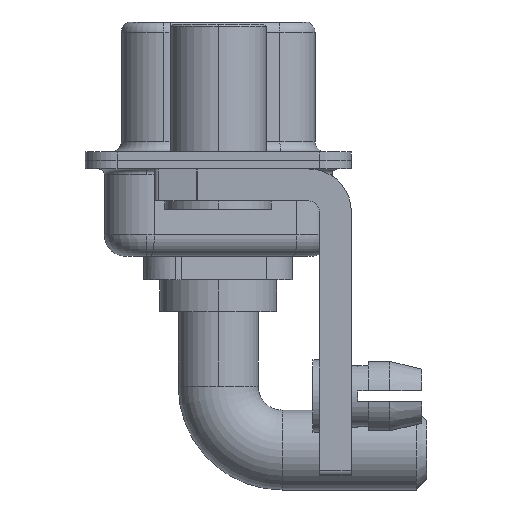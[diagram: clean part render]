
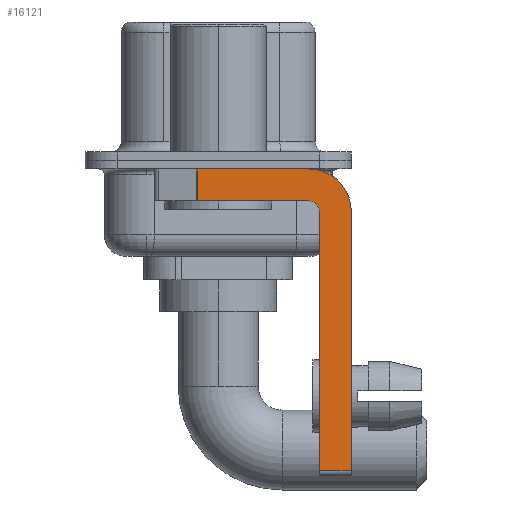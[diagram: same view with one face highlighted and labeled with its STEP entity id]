
A CAD part, left-side view. The second image highlights one B-rep face of the part: STEP entity #16121.
In plain terms, the highlighted planar face has unit normal (-1, 0, 0).
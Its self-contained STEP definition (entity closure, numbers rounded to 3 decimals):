
#6 = ORIENTED_EDGE ( 'NONE', *, *, #10254, .T. ) ;
#32 = CARTESIAN_POINT ( 'NONE',  ( -2.9, 3., -0.4 ) ) ;
#87 = EDGE_CURVE ( 'NONE', #12321, #15476, #3806, .T. ) ;
#137 = DIRECTION ( 'NONE',  ( 0., -1., 0. ) ) ;
#164 = CARTESIAN_POINT ( 'NONE',  ( -2.9, -4.25, -2.4 ) ) ;
#516 = LINE ( 'NONE', #9649, #14072 ) ;
#569 = VECTOR ( 'NONE', #2551, 1000. ) ;
#1224 = EDGE_CURVE ( 'NONE', #12321, #5367, #13793, .T. ) ;
#1238 = VERTEX_POINT ( 'NONE', #9274 ) ;
#2274 = ORIENTED_EDGE ( 'NONE', *, *, #1224, .F. ) ;
#2551 = DIRECTION ( 'NONE',  ( 0., 0., -1. ) ) ;
#2997 = CARTESIAN_POINT ( 'NONE',  ( -2.9, -4.25, -2.4 ) ) ;
#3165 = DIRECTION ( 'NONE',  ( 0., 0., -1. ) ) ;
#3273 = EDGE_CURVE ( 'NONE', #15212, #1238, #5112, .T. ) ;
#3745 = VECTOR ( 'NONE', #6635, 1000. ) ;
#3806 = LINE ( 'NONE', #11234, #10493 ) ;
#4442 = VECTOR ( 'NONE', #137, 1000. ) ;
#4486 = CARTESIAN_POINT ( 'NONE',  ( -2.9, -4.75, -14.8 ) ) ;
#4522 = CARTESIAN_POINT ( 'NONE',  ( -2.9, -4.75, -14.55 ) ) ;
#5112 = CIRCLE ( 'NONE', #16330, 0.5 ) ;
#5367 = VERTEX_POINT ( 'NONE', #14962 ) ;
#5429 = FACE_OUTER_BOUND ( 'NONE', #17539, .T. ) ;
#5823 = ORIENTED_EDGE ( 'NONE', *, *, #3273, .F. ) ;
#5919 = DIRECTION ( 'NONE',  ( -1., 0., 0. ) ) ;
#6004 = VERTEX_POINT ( 'NONE', #9235 ) ;
#6635 = DIRECTION ( 'NONE',  ( 0., -1., 0. ) ) ;
#7605 = DIRECTION ( 'NONE',  ( 0., 0., 1. ) ) ;
#8088 = ORIENTED_EDGE ( 'NONE', *, *, #14911, .F. ) ;
#8752 = CARTESIAN_POINT ( 'NONE',  ( -2.9, -4.25, -2.4 ) ) ;
#8936 = PLANE ( 'NONE',  #19834 ) ;
#9235 = CARTESIAN_POINT ( 'NONE',  ( -2.9, -6.25, -14.55 ) ) ;
#9274 = CARTESIAN_POINT ( 'NONE',  ( -2.9, -4.25, -1.9 ) ) ;
#9329 = CARTESIAN_POINT ( 'NONE',  ( -2.9, -6.25, -2.4 ) ) ;
#9649 = CARTESIAN_POINT ( 'NONE',  ( -2.9, -4.25, -1.9 ) ) ;
#9940 = DIRECTION ( 'NONE',  ( 0., 0., -1. ) ) ;
#10063 = CIRCLE ( 'NONE', #16140, 2. ) ;
#10254 = EDGE_CURVE ( 'NONE', #14788, #6004, #17250, .T. ) ;
#10441 = VERTEX_POINT ( 'NONE', #9329 ) ;
#10493 = VECTOR ( 'NONE', #9940, 1000. ) ;
#10793 = CARTESIAN_POINT ( 'NONE',  ( -2.9, 0.978, -0.4 ) ) ;
#10906 = ORIENTED_EDGE ( 'NONE', *, *, #12339, .F. ) ;
#11234 = CARTESIAN_POINT ( 'NONE',  ( -2.9, 0.978, -1.9 ) ) ;
#12126 = DIRECTION ( 'NONE',  ( 0., 0., 1. ) ) ;
#12321 = VERTEX_POINT ( 'NONE', #10793 ) ;
#12339 = EDGE_CURVE ( 'NONE', #5367, #10441, #10063, .T. ) ;
#13454 = DIRECTION ( 'NONE',  ( 1., 0., 0. ) ) ;
#13474 = EDGE_CURVE ( 'NONE', #14788, #15212, #19729, .T. ) ;
#13708 = CARTESIAN_POINT ( 'NONE',  ( -2.9, -4.75, -2.4 ) ) ;
#13793 = LINE ( 'NONE', #32, #4442 ) ;
#14072 = VECTOR ( 'NONE', #15761, 1000. ) ;
#14200 = EDGE_CURVE ( 'NONE', #10441, #6004, #19102, .T. ) ;
#14706 = CARTESIAN_POINT ( 'NONE',  ( -2.9, -6.25, -2.4 ) ) ;
#14788 = VERTEX_POINT ( 'NONE', #4522 ) ;
#14911 = EDGE_CURVE ( 'NONE', #1238, #15476, #516, .T. ) ;
#14962 = CARTESIAN_POINT ( 'NONE',  ( -2.9, -4.25, -0.4 ) ) ;
#15212 = VERTEX_POINT ( 'NONE', #13708 ) ;
#15476 = VERTEX_POINT ( 'NONE', #16499 ) ;
#15761 = DIRECTION ( 'NONE',  ( 0., 1., 0. ) ) ;
#15929 = VECTOR ( 'NONE', #7605, 1000. ) ;
#16121 = ADVANCED_FACE ( 'NONE', ( #5429 ), #8936, .F. ) ;
#16140 = AXIS2_PLACEMENT_3D ( 'NONE', #164, #16911, #3165 ) ;
#16330 = AXIS2_PLACEMENT_3D ( 'NONE', #2997, #5919, #12126 ) ;
#16499 = CARTESIAN_POINT ( 'NONE',  ( -2.9, 0.978, -1.9 ) ) ;
#16735 = ORIENTED_EDGE ( 'NONE', *, *, #87, .T. ) ;
#16911 = DIRECTION ( 'NONE',  ( 1., 0., 0. ) ) ;
#17250 = LINE ( 'NONE', #17354, #3745 ) ;
#17354 = CARTESIAN_POINT ( 'NONE',  ( -2.9, -4.25, -14.55 ) ) ;
#17539 = EDGE_LOOP ( 'NONE', ( #2274, #16735, #8088, #5823, #18178, #6, #19484, #10906 ) ) ;
#18178 = ORIENTED_EDGE ( 'NONE', *, *, #13474, .F. ) ;
#19102 = LINE ( 'NONE', #14706, #569 ) ;
#19484 = ORIENTED_EDGE ( 'NONE', *, *, #14200, .F. ) ;
#19547 = DIRECTION ( 'NONE',  ( 0., 0., -1. ) ) ;
#19729 = LINE ( 'NONE', #4486, #15929 ) ;
#19834 = AXIS2_PLACEMENT_3D ( 'NONE', #8752, #13454, #19547 ) ;
